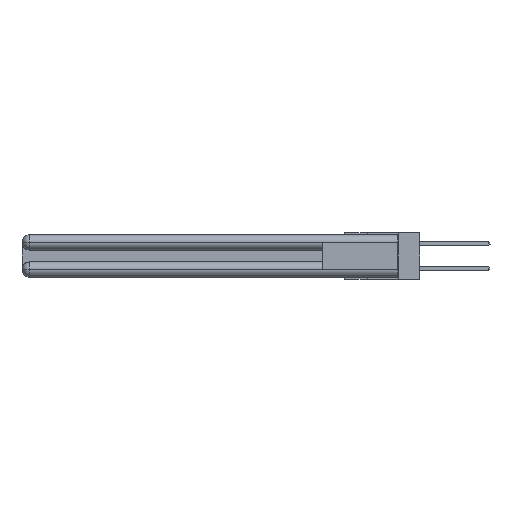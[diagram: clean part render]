
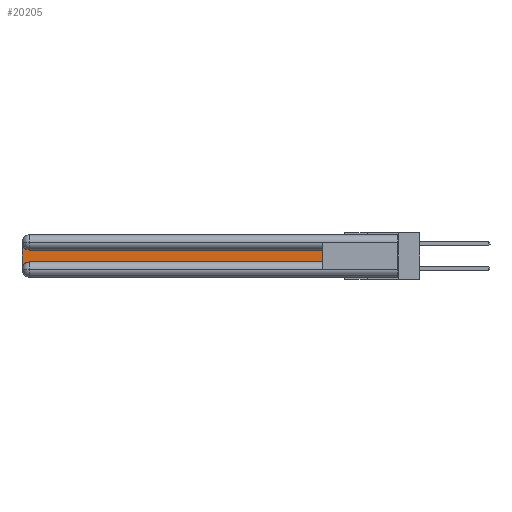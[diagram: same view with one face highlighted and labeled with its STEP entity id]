
A CAD part, left-side view. The second image highlights one B-rep face of the part: STEP entity #20205.
In plain terms, the highlighted planar face has unit normal (-1, 0, 0).
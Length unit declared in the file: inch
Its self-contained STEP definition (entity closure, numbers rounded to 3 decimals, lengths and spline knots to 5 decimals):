
#1922 = CARTESIAN_POINT ( 'NONE',  ( 0.075, 2.94, -0.2175 ) ) ;
#2062 = EDGE_CURVE ( 'NONE', #3385, #32528, #17707, .T. ) ;
#2076 = ORIENTED_EDGE ( 'NONE', *, *, #6251, .T. ) ;
#3385 = VERTEX_POINT ( 'NONE', #27414 ) ;
#3489 = VECTOR ( 'NONE', #17635, 39.37008 ) ;
#4661 = DIRECTION ( 'NONE',  ( 0., 0., -1. ) ) ;
#4677 = VECTOR ( 'NONE', #22637, 39.37008 ) ;
#4877 = DIRECTION ( 'NONE',  ( 0., 0., -1. ) ) ;
#5617 = VECTOR ( 'NONE', #4661, 39.37008 ) ;
#6036 = CARTESIAN_POINT ( 'NONE',  ( 0.075, 3., -0.0625 ) ) ;
#6251 = EDGE_CURVE ( 'NONE', #20928, #23474, #12748, .T. ) ;
#6734 = CARTESIAN_POINT ( 'NONE',  ( 0.075, 2.94, -0.2775 ) ) ;
#6944 = DIRECTION ( 'NONE',  ( 1., 0., 0. ) ) ;
#7277 = CARTESIAN_POINT ( 'NONE',  ( 0.075, 0.6, -0.1225 ) ) ;
#7662 = CARTESIAN_POINT ( 'NONE',  ( 0.075, 0.6, -0.2175 ) ) ;
#7700 = EDGE_CURVE ( 'NONE', #32528, #16040, #28147, .T. ) ;
#9393 = VERTEX_POINT ( 'NONE', #6036 ) ;
#11949 = CARTESIAN_POINT ( 'NONE',  ( 0.075, 3., -0.1225 ) ) ;
#12007 = DIRECTION ( 'NONE',  ( 0., 0., -1. ) ) ;
#12748 = CIRCLE ( 'NONE', #25868, 0.06 ) ;
#12987 = DIRECTION ( 'NONE',  ( 1., 0., 0. ) ) ;
#13137 = LINE ( 'NONE', #16836, #5617 ) ;
#13476 = VECTOR ( 'NONE', #27920, 39.37008 ) ;
#13525 = EDGE_LOOP ( 'NONE', ( #14180, #30294, #31322, #2076, #28534, #18893 ) ) ;
#14180 = ORIENTED_EDGE ( 'NONE', *, *, #7700, .T. ) ;
#16040 = VERTEX_POINT ( 'NONE', #28181 ) ;
#16836 = CARTESIAN_POINT ( 'NONE',  ( 0.075, 3., -0.2175 ) ) ;
#17287 = AXIS2_PLACEMENT_3D ( 'NONE', #28189, #12987, #4877 ) ;
#17635 = DIRECTION ( 'NONE',  ( 0., 0., 1. ) ) ;
#17707 = LINE ( 'NONE', #29992, #3489 ) ;
#18893 = ORIENTED_EDGE ( 'NONE', *, *, #2062, .T. ) ;
#18989 = LINE ( 'NONE', #7662, #13476 ) ;
#19138 = CIRCLE ( 'NONE', #17287, 0.06 ) ;
#19676 = AXIS2_PLACEMENT_3D ( 'NONE', #11949, #21770, #32032 ) ;
#20205 = ADVANCED_FACE ( 'NONE', ( #25611 ), #27036, .F. ) ;
#20928 = VERTEX_POINT ( 'NONE', #30564 ) ;
#21770 = DIRECTION ( 'NONE',  ( 1., 0., 0. ) ) ;
#22637 = DIRECTION ( 'NONE',  ( 0., 1., 0. ) ) ;
#23474 = VERTEX_POINT ( 'NONE', #1922 ) ;
#23972 = EDGE_CURVE ( 'NONE', #9393, #20928, #13137, .T. ) ;
#25611 = FACE_OUTER_BOUND ( 'NONE', #13525, .T. ) ;
#25868 = AXIS2_PLACEMENT_3D ( 'NONE', #6734, #6944, #12007 ) ;
#26848 = EDGE_CURVE ( 'NONE', #23474, #3385, #18989, .T. ) ;
#27036 = PLANE ( 'NONE',  #19676 ) ;
#27414 = CARTESIAN_POINT ( 'NONE',  ( 0.075, 0.6, -0.2175 ) ) ;
#27920 = DIRECTION ( 'NONE',  ( 0., -1., 0. ) ) ;
#28147 = LINE ( 'NONE', #7277, #4677 ) ;
#28181 = CARTESIAN_POINT ( 'NONE',  ( 0.075, 2.94, -0.1225 ) ) ;
#28189 = CARTESIAN_POINT ( 'NONE',  ( 0.075, 2.94, -0.0625 ) ) ;
#28534 = ORIENTED_EDGE ( 'NONE', *, *, #26848, .T. ) ;
#29992 = CARTESIAN_POINT ( 'NONE',  ( 0.075, 0.6, -0.2175 ) ) ;
#30294 = ORIENTED_EDGE ( 'NONE', *, *, #31575, .T. ) ;
#30564 = CARTESIAN_POINT ( 'NONE',  ( 0.075, 3., -0.2775 ) ) ;
#31122 = CARTESIAN_POINT ( 'NONE',  ( 0.075, 0.6, -0.1225 ) ) ;
#31322 = ORIENTED_EDGE ( 'NONE', *, *, #23972, .T. ) ;
#31575 = EDGE_CURVE ( 'NONE', #16040, #9393, #19138, .T. ) ;
#32032 = DIRECTION ( 'NONE',  ( 0., 0., -1. ) ) ;
#32528 = VERTEX_POINT ( 'NONE', #31122 ) ;
